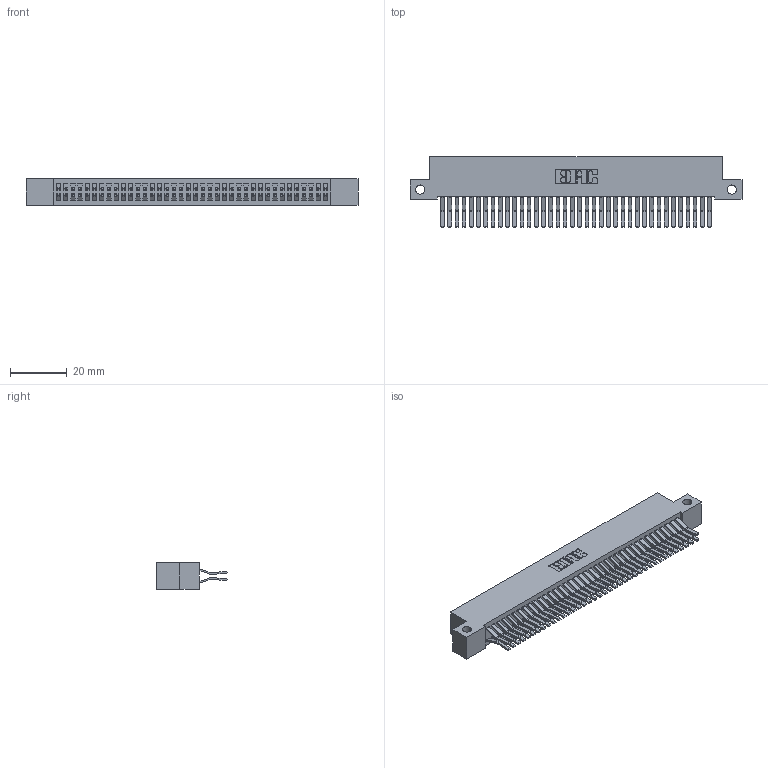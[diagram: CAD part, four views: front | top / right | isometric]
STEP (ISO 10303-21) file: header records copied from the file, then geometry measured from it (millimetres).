
FILE_DESCRIPTION (( 'STEP AP203' ), '1' );
FILE_NAME ('392-076-560-212.STEP', '2018-08-18T01:53:44', ( '' ), ( '' ), 'SwSTEP 2.0', 'SolidWorks 2016', '' );
FILE_SCHEMA (( 'CONFIG_CONTROL_DESIGN' ));
Length unit declared in the file: inch
Products named in the file (3): 342 Part_Side Mount; 345-292-001_560 Tail; 392-076-560-212
Assembly tree (77 placements, depth 2):
  392-076-560-212
    342 Part_Side Mount
    345-292-001_560 Tail  x76
Bounding box: 116.84 x 24.78 x 9.4 mm (x, y, z)
Volume: 10904.2 mm3; surface area: 18687.4 mm2
Topology: 77 solids, 77 shells, 4214 faces, 12535 edges, 8254 vertices
Faces by surface type: plane 2802, cylinder 1412
Entity records: 24923 total; most frequent: CARTESIAN_POINT 4134, ORIENTED_EDGE 4070, DIRECTION 3543, EDGE_CURVE 2035, VECTOR 1903, LINE 1903, VERTEX_POINT 1354, AXIS2_PLACEMENT_3D 820
